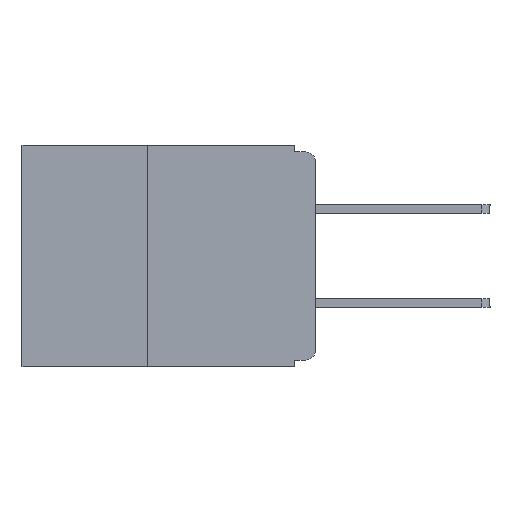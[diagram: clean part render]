
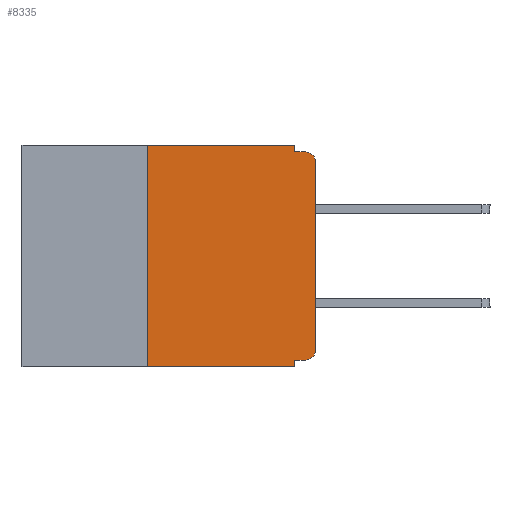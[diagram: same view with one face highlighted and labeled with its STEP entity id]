
A CAD part, left-side view. The second image highlights one B-rep face of the part: STEP entity #8335.
In plain terms, the highlighted planar face has unit normal (-1, 0, 0).
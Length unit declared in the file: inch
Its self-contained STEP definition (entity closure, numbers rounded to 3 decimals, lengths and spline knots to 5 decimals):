
#45 = ORIENTED_EDGE ( 'NONE', *, *, #8196, .F. ) ;
#49 = CARTESIAN_POINT ( 'NONE',  ( 0., 0.031, 0. ) ) ;
#185 = DIRECTION ( 'NONE',  ( 0., 0., -1. ) ) ;
#328 = LINE ( 'NONE', #8227, #6856 ) ;
#369 = VERTEX_POINT ( 'NONE', #49 ) ;
#630 = CARTESIAN_POINT ( 'NONE',  ( 0., 0., 0. ) ) ;
#663 = ORIENTED_EDGE ( 'NONE', *, *, #12773, .F. ) ;
#695 = VECTOR ( 'NONE', #13075, 39.37008 ) ;
#864 = VERTEX_POINT ( 'NONE', #13674 ) ;
#1062 = ORIENTED_EDGE ( 'NONE', *, *, #11018, .T. ) ;
#1239 = LINE ( 'NONE', #8012, #7331 ) ;
#1281 = CARTESIAN_POINT ( 'NONE',  ( 0., 0.015, -0.025 ) ) ;
#1292 = DIRECTION ( 'NONE',  ( 0., -1., 0. ) ) ;
#1374 = CARTESIAN_POINT ( 'NONE',  ( 0., 0.25, -0.33 ) ) ;
#1622 = DIRECTION ( 'NONE',  ( 0., 0., -1. ) ) ;
#2187 = EDGE_CURVE ( 'NONE', #864, #8132, #13663, .T. ) ;
#2339 = VERTEX_POINT ( 'NONE', #5067 ) ;
#2453 = LINE ( 'NONE', #12272, #5008 ) ;
#2578 = AXIS2_PLACEMENT_3D ( 'NONE', #13516, #8811, #1622 ) ;
#2990 = EDGE_CURVE ( 'NONE', #369, #14260, #328, .T. ) ;
#3195 = DIRECTION ( 'NONE',  ( 0., 0., 1. ) ) ;
#3444 = ORIENTED_EDGE ( 'NONE', *, *, #4267, .F. ) ;
#3644 = ORIENTED_EDGE ( 'NONE', *, *, #4748, .F. ) ;
#3745 = VERTEX_POINT ( 'NONE', #10232 ) ;
#4128 = ORIENTED_EDGE ( 'NONE', *, *, #12354, .T. ) ;
#4267 = EDGE_CURVE ( 'NONE', #10121, #3745, #2453, .T. ) ;
#4268 = VECTOR ( 'NONE', #9013, 39.37008 ) ;
#4748 = EDGE_CURVE ( 'NONE', #7803, #10121, #8079, .T. ) ;
#4821 = CARTESIAN_POINT ( 'NONE',  ( 0., 0.031, -0.01 ) ) ;
#4953 = CARTESIAN_POINT ( 'NONE',  ( 0., 0., -0.32 ) ) ;
#4974 = CARTESIAN_POINT ( 'NONE',  ( 0., 0.015, -0.305 ) ) ;
#5008 = VECTOR ( 'NONE', #5280, 39.37008 ) ;
#5067 = CARTESIAN_POINT ( 'NONE',  ( 0., 0.25, 0. ) ) ;
#5277 = PLANE ( 'NONE',  #2578 ) ;
#5278 = FACE_OUTER_BOUND ( 'NONE', #6324, .T. ) ;
#5280 = DIRECTION ( 'NONE',  ( 0., 0., -1. ) ) ;
#6052 = CARTESIAN_POINT ( 'NONE',  ( 0., 0.437, -0.33 ) ) ;
#6132 = DIRECTION ( 'NONE',  ( 0., 0., -1. ) ) ;
#6182 = CARTESIAN_POINT ( 'NONE',  ( 0., 0.437, 0. ) ) ;
#6324 = EDGE_LOOP ( 'NONE', ( #8658, #8394, #8141, #7770, #45, #663, #1062, #3444, #3644, #4128 ) ) ;
#6376 = VECTOR ( 'NONE', #1292, 39.37008 ) ;
#6634 = CIRCLE ( 'NONE', #14579, 0.015 ) ;
#6856 = VECTOR ( 'NONE', #8157, 39.37008 ) ;
#7331 = VECTOR ( 'NONE', #9137, 39.37008 ) ;
#7565 = CARTESIAN_POINT ( 'NONE',  ( 0., 0.015, -0.32 ) ) ;
#7770 = ORIENTED_EDGE ( 'NONE', *, *, #2990, .F. ) ;
#7803 = VERTEX_POINT ( 'NONE', #7565 ) ;
#8012 = CARTESIAN_POINT ( 'NONE',  ( 0., 0.25, -0.33 ) ) ;
#8079 = LINE ( 'NONE', #4953, #10464 ) ;
#8132 = VERTEX_POINT ( 'NONE', #10778 ) ;
#8141 = ORIENTED_EDGE ( 'NONE', *, *, #10745, .F. ) ;
#8157 = DIRECTION ( 'NONE',  ( 0., 0., -1. ) ) ;
#8196 = EDGE_CURVE ( 'NONE', #2339, #369, #9457, .T. ) ;
#8227 = CARTESIAN_POINT ( 'NONE',  ( 0., 0.031, 0. ) ) ;
#8335 = ADVANCED_FACE ( 'NONE', ( #5278 ), #5277, .F. ) ;
#8394 = ORIENTED_EDGE ( 'NONE', *, *, #2187, .T. ) ;
#8658 = ORIENTED_EDGE ( 'NONE', *, *, #14631, .T. ) ;
#8811 = DIRECTION ( 'NONE',  ( 1., 0., 0. ) ) ;
#8851 = VECTOR ( 'NONE', #3195, 39.37008 ) ;
#9013 = DIRECTION ( 'NONE',  ( 0., -1., 0. ) ) ;
#9137 = DIRECTION ( 'NONE',  ( 0., 0., 1. ) ) ;
#9457 = LINE ( 'NONE', #6182, #6376 ) ;
#10121 = VERTEX_POINT ( 'NONE', #11384 ) ;
#10232 = CARTESIAN_POINT ( 'NONE',  ( 0., 0.031, -0.33 ) ) ;
#10464 = VECTOR ( 'NONE', #14287, 39.37008 ) ;
#10480 = LINE ( 'NONE', #14757, #4268 ) ;
#10745 = EDGE_CURVE ( 'NONE', #14260, #8132, #10480, .T. ) ;
#10778 = CARTESIAN_POINT ( 'NONE',  ( 0., 0.015, -0.01 ) ) ;
#11018 = EDGE_CURVE ( 'NONE', #11163, #3745, #13051, .T. ) ;
#11163 = VERTEX_POINT ( 'NONE', #1374 ) ;
#11384 = CARTESIAN_POINT ( 'NONE',  ( 0., 0.031, -0.32 ) ) ;
#11623 = AXIS2_PLACEMENT_3D ( 'NONE', #1281, #15353, #185 ) ;
#11978 = LINE ( 'NONE', #630, #8851 ) ;
#12272 = CARTESIAN_POINT ( 'NONE',  ( 0., 0.031, -0.33 ) ) ;
#12354 = EDGE_CURVE ( 'NONE', #7803, #13527, #6634, .T. ) ;
#12773 = EDGE_CURVE ( 'NONE', #11163, #2339, #1239, .T. ) ;
#13051 = LINE ( 'NONE', #6052, #695 ) ;
#13075 = DIRECTION ( 'NONE',  ( 0., -1., 0. ) ) ;
#13155 = DIRECTION ( 'NONE',  ( -1., 0., 0. ) ) ;
#13516 = CARTESIAN_POINT ( 'NONE',  ( 0., 0.437, 0. ) ) ;
#13527 = VERTEX_POINT ( 'NONE', #14053 ) ;
#13663 = CIRCLE ( 'NONE', #11623, 0.015 ) ;
#13674 = CARTESIAN_POINT ( 'NONE',  ( 0., 0., -0.025 ) ) ;
#14053 = CARTESIAN_POINT ( 'NONE',  ( 0., 0., -0.305 ) ) ;
#14260 = VERTEX_POINT ( 'NONE', #4821 ) ;
#14287 = DIRECTION ( 'NONE',  ( 0., 1., 0. ) ) ;
#14579 = AXIS2_PLACEMENT_3D ( 'NONE', #4974, #13155, #6132 ) ;
#14631 = EDGE_CURVE ( 'NONE', #13527, #864, #11978, .T. ) ;
#14757 = CARTESIAN_POINT ( 'NONE',  ( 0., 0., -0.01 ) ) ;
#15353 = DIRECTION ( 'NONE',  ( -1., 0., 0. ) ) ;
